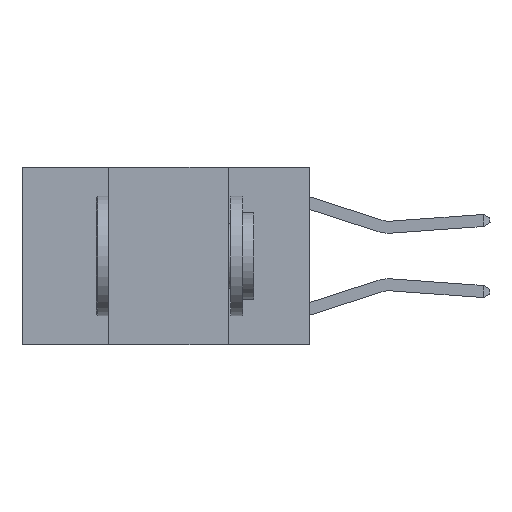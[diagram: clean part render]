
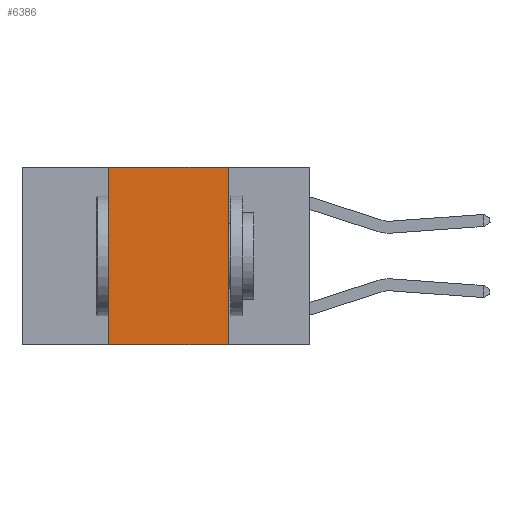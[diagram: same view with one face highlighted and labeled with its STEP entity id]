
A CAD part, left-side view. The second image highlights one B-rep face of the part: STEP entity #6386.
In plain terms, the highlighted planar face has unit normal (-1, 0, 0).
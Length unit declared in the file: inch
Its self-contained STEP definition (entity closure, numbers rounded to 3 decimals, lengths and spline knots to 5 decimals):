
#79 = VERTEX_POINT ( 'NONE', #3618 ) ;
#663 = CARTESIAN_POINT ( 'NONE',  ( 0., 0.42, -0.37 ) ) ;
#1137 = DIRECTION ( 'NONE',  ( 0., -1., 0. ) ) ;
#1158 = EDGE_CURVE ( 'NONE', #5896, #3820, #10505, .T. ) ;
#1277 = EDGE_CURVE ( 'NONE', #5929, #79, #4794, .T. ) ;
#1881 = VECTOR ( 'NONE', #3802, 39.37008 ) ;
#1913 = CARTESIAN_POINT ( 'NONE',  ( 0., 0.42, 0. ) ) ;
#2399 = EDGE_CURVE ( 'NONE', #5929, #3820, #9950, .T. ) ;
#2534 = DIRECTION ( 'NONE',  ( 0., -1., 0. ) ) ;
#3091 = CARTESIAN_POINT ( 'NONE',  ( 0., 0.6, 0. ) ) ;
#3618 = CARTESIAN_POINT ( 'NONE',  ( 0., 0.42, 0. ) ) ;
#3802 = DIRECTION ( 'NONE',  ( 0., 0., -1. ) ) ;
#3820 = VERTEX_POINT ( 'NONE', #3864 ) ;
#3864 = CARTESIAN_POINT ( 'NONE',  ( 0., 0.17, -0.37 ) ) ;
#3975 = PLANE ( 'NONE',  #7596 ) ;
#4002 = VECTOR ( 'NONE', #2534, 39.37008 ) ;
#4785 = DIRECTION ( 'NONE',  ( 1., 0., 0. ) ) ;
#4794 = LINE ( 'NONE', #1913, #6301 ) ;
#5128 = DIRECTION ( 'NONE',  ( 0., 0., 1. ) ) ;
#5560 = VECTOR ( 'NONE', #1137, 39.37008 ) ;
#5896 = VERTEX_POINT ( 'NONE', #9812 ) ;
#5929 = VERTEX_POINT ( 'NONE', #663 ) ;
#6069 = EDGE_LOOP ( 'NONE', ( #9100, #6656, #7824, #7107 ) ) ;
#6158 = CARTESIAN_POINT ( 'NONE',  ( 0., 0.17, 0. ) ) ;
#6301 = VECTOR ( 'NONE', #5128, 39.37008 ) ;
#6386 = ADVANCED_FACE ( 'NONE', ( #8969 ), #3975, .F. ) ;
#6656 = ORIENTED_EDGE ( 'NONE', *, *, #8162, .F. ) ;
#7107 = ORIENTED_EDGE ( 'NONE', *, *, #2399, .T. ) ;
#7167 = CARTESIAN_POINT ( 'NONE',  ( 0., 0.6, -0.37 ) ) ;
#7596 = AXIS2_PLACEMENT_3D ( 'NONE', #3091, #4785, #10356 ) ;
#7824 = ORIENTED_EDGE ( 'NONE', *, *, #1277, .F. ) ;
#8162 = EDGE_CURVE ( 'NONE', #79, #5896, #8378, .T. ) ;
#8378 = LINE ( 'NONE', #9142, #4002 ) ;
#8969 = FACE_OUTER_BOUND ( 'NONE', #6069, .T. ) ;
#9100 = ORIENTED_EDGE ( 'NONE', *, *, #1158, .F. ) ;
#9142 = CARTESIAN_POINT ( 'NONE',  ( 0., 0.6, 0. ) ) ;
#9812 = CARTESIAN_POINT ( 'NONE',  ( 0., 0.17, 0. ) ) ;
#9950 = LINE ( 'NONE', #7167, #5560 ) ;
#10356 = DIRECTION ( 'NONE',  ( 0., 0., -1. ) ) ;
#10505 = LINE ( 'NONE', #6158, #1881 ) ;
